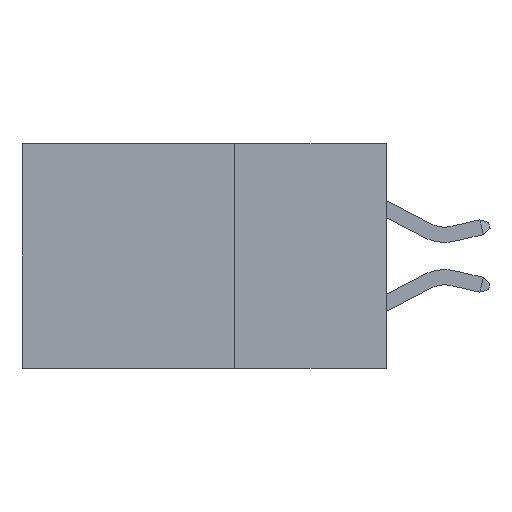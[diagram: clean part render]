
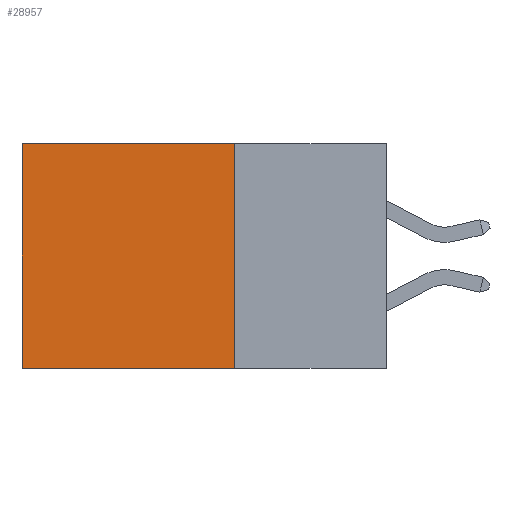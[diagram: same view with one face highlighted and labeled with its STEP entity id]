
A CAD part, left-side view. The second image highlights one B-rep face of the part: STEP entity #28957.
In plain terms, the highlighted planar face has unit normal (-1, 0, 0).
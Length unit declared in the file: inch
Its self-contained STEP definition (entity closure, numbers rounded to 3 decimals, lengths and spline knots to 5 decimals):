
#513 = PLANE ( 'NONE',  #1041 ) ;
#574 = CARTESIAN_POINT ( 'NONE',  ( 0.298, 0.6, 0. ) ) ;
#1041 = AXIS2_PLACEMENT_3D ( 'NONE', #18337, #13064, #26033 ) ;
#1452 = VERTEX_POINT ( 'NONE', #20612 ) ;
#2300 = ORIENTED_EDGE ( 'NONE', *, *, #32731, .T. ) ;
#3532 = CARTESIAN_POINT ( 'NONE',  ( 0.298, 0.25, -0.37 ) ) ;
#4044 = CARTESIAN_POINT ( 'NONE',  ( 0.298, 0.25, 0. ) ) ;
#5268 = EDGE_CURVE ( 'NONE', #12947, #10549, #27510, .T. ) ;
#5349 = VECTOR ( 'NONE', #20915, 39.37008 ) ;
#7718 = LINE ( 'NONE', #574, #10459 ) ;
#8940 = DIRECTION ( 'NONE',  ( 0., 1., 0. ) ) ;
#10459 = VECTOR ( 'NONE', #31028, 39.37008 ) ;
#10549 = VERTEX_POINT ( 'NONE', #16177 ) ;
#10974 = CARTESIAN_POINT ( 'NONE',  ( 0.298, 0.25, -0.37 ) ) ;
#12947 = VERTEX_POINT ( 'NONE', #4044 ) ;
#13064 = DIRECTION ( 'NONE',  ( 1., 0., 0. ) ) ;
#13084 = VERTEX_POINT ( 'NONE', #10974 ) ;
#13796 = LINE ( 'NONE', #29063, #32014 ) ;
#16177 = CARTESIAN_POINT ( 'NONE',  ( 0.298, 0.6, 0. ) ) ;
#17082 = FACE_OUTER_BOUND ( 'NONE', #30980, .T. ) ;
#18337 = CARTESIAN_POINT ( 'NONE',  ( 0.298, 0.25, 0. ) ) ;
#20612 = CARTESIAN_POINT ( 'NONE',  ( 0.298, 0.6, -0.37 ) ) ;
#20915 = DIRECTION ( 'NONE',  ( 0., 1., 0. ) ) ;
#21027 = CARTESIAN_POINT ( 'NONE',  ( 0.298, 0.25, 0. ) ) ;
#21143 = ORIENTED_EDGE ( 'NONE', *, *, #5268, .T. ) ;
#22134 = EDGE_CURVE ( 'NONE', #13084, #1452, #31628, .T. ) ;
#22626 = EDGE_CURVE ( 'NONE', #12947, #13084, #13796, .T. ) ;
#22915 = ORIENTED_EDGE ( 'NONE', *, *, #22134, .F. ) ;
#25528 = ORIENTED_EDGE ( 'NONE', *, *, #22626, .F. ) ;
#26033 = DIRECTION ( 'NONE',  ( 0., 0., -1. ) ) ;
#27510 = LINE ( 'NONE', #21027, #5349 ) ;
#27682 = VECTOR ( 'NONE', #8940, 39.37008 ) ;
#28957 = ADVANCED_FACE ( 'NONE', ( #17082 ), #513, .F. ) ;
#29063 = CARTESIAN_POINT ( 'NONE',  ( 0.298, 0.25, 0. ) ) ;
#29271 = DIRECTION ( 'NONE',  ( 0., 0., -1. ) ) ;
#30980 = EDGE_LOOP ( 'NONE', ( #2300, #22915, #25528, #21143 ) ) ;
#31028 = DIRECTION ( 'NONE',  ( 0., 0., -1. ) ) ;
#31628 = LINE ( 'NONE', #3532, #27682 ) ;
#32014 = VECTOR ( 'NONE', #29271, 39.37008 ) ;
#32731 = EDGE_CURVE ( 'NONE', #10549, #1452, #7718, .T. ) ;
